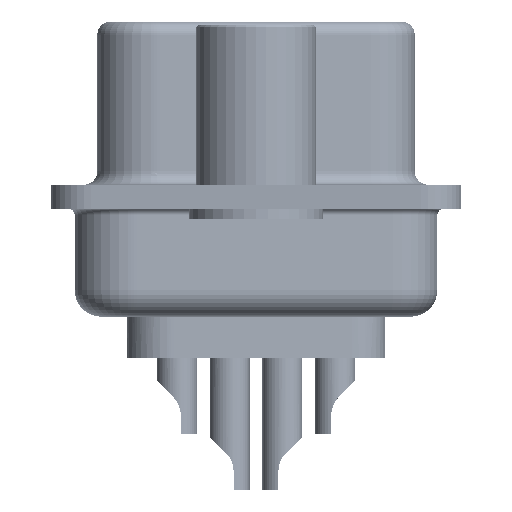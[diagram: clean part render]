
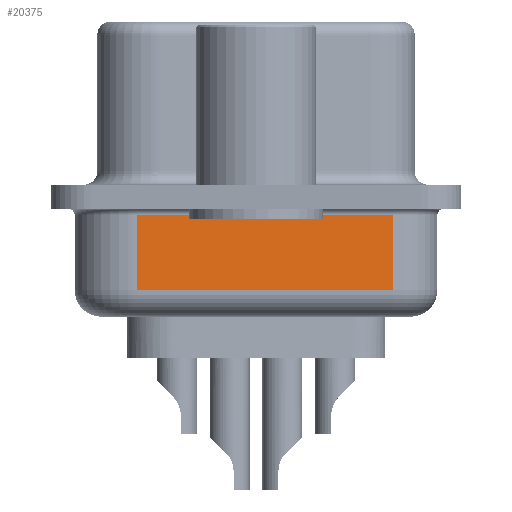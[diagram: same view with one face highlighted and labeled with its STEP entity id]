
A CAD part, left-side view. The second image highlights one B-rep face of the part: STEP entity #20375.
In plain terms, the highlighted planar face has unit normal (-0.985, -0.174, 0).
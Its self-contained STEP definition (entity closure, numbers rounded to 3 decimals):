
#343 = LINE ( 'NONE', #9798, #8146 ) ;
#2232 = EDGE_CURVE ( 'NONE', #6393, #16421, #13125, .T. ) ;
#4731 = CARTESIAN_POINT ( 'NONE',  ( 3.03, 4.453, -0.7 ) ) ;
#5088 = PLANE ( 'NONE',  #23335 ) ;
#5154 = DIRECTION ( 'NONE',  ( -0.174, 0.985, 0. ) ) ;
#6393 = VERTEX_POINT ( 'NONE', #30864 ) ;
#7155 = VERTEX_POINT ( 'NONE', #12747 ) ;
#8146 = VECTOR ( 'NONE', #29560, 1000. ) ;
#9311 = VERTEX_POINT ( 'NONE', #39427 ) ;
#9707 = DIRECTION ( 'NONE',  ( 0., 0., 1. ) ) ;
#9798 = CARTESIAN_POINT ( 'NONE',  ( 3.03, 4.453, -3.5 ) ) ;
#12747 = CARTESIAN_POINT ( 'NONE',  ( 3.03, 4.453, -0.7 ) ) ;
#13125 = LINE ( 'NONE', #13760, #29539 ) ;
#13760 = CARTESIAN_POINT ( 'NONE',  ( 4.723, -5.147, -4.5 ) ) ;
#15387 = EDGE_CURVE ( 'NONE', #9311, #7155, #37849, .T. ) ;
#16421 = VERTEX_POINT ( 'NONE', #24924 ) ;
#17728 = DIRECTION ( 'NONE',  ( 0.985, 0.174, 0. ) ) ;
#18074 = VECTOR ( 'NONE', #5154, 1000. ) ;
#18179 = EDGE_CURVE ( 'NONE', #16421, #7155, #26475, .T. ) ;
#18495 = DIRECTION ( 'NONE',  ( 0., 0., 1. ) ) ;
#20375 = ADVANCED_FACE ( 'NONE', ( #27630 ), #5088, .F. ) ;
#23335 = AXIS2_PLACEMENT_3D ( 'NONE', #23762, #17728, #24180 ) ;
#23762 = CARTESIAN_POINT ( 'NONE',  ( 3.03, 4.453, -4.5 ) ) ;
#24180 = DIRECTION ( 'NONE',  ( -0.174, 0.985, 0. ) ) ;
#24924 = CARTESIAN_POINT ( 'NONE',  ( 4.723, -5.147, -0.7 ) ) ;
#25858 = ORIENTED_EDGE ( 'NONE', *, *, #2232, .T. ) ;
#26475 = LINE ( 'NONE', #4731, #18074 ) ;
#27630 = FACE_OUTER_BOUND ( 'NONE', #35817, .T. ) ;
#29539 = VECTOR ( 'NONE', #9707, 1000. ) ;
#29560 = DIRECTION ( 'NONE',  ( 0.174, -0.985, 0. ) ) ;
#30864 = CARTESIAN_POINT ( 'NONE',  ( 4.723, -5.147, -3.5 ) ) ;
#33105 = VECTOR ( 'NONE', #18495, 1000. ) ;
#34055 = ORIENTED_EDGE ( 'NONE', *, *, #18179, .T. ) ;
#35066 = CARTESIAN_POINT ( 'NONE',  ( 3.03, 4.453, -4.5 ) ) ;
#35817 = EDGE_LOOP ( 'NONE', ( #36141, #40587, #25858, #34055 ) ) ;
#36141 = ORIENTED_EDGE ( 'NONE', *, *, #15387, .F. ) ;
#37849 = LINE ( 'NONE', #35066, #33105 ) ;
#39427 = CARTESIAN_POINT ( 'NONE',  ( 3.03, 4.453, -3.5 ) ) ;
#39448 = EDGE_CURVE ( 'NONE', #9311, #6393, #343, .T. ) ;
#40587 = ORIENTED_EDGE ( 'NONE', *, *, #39448, .T. ) ;
